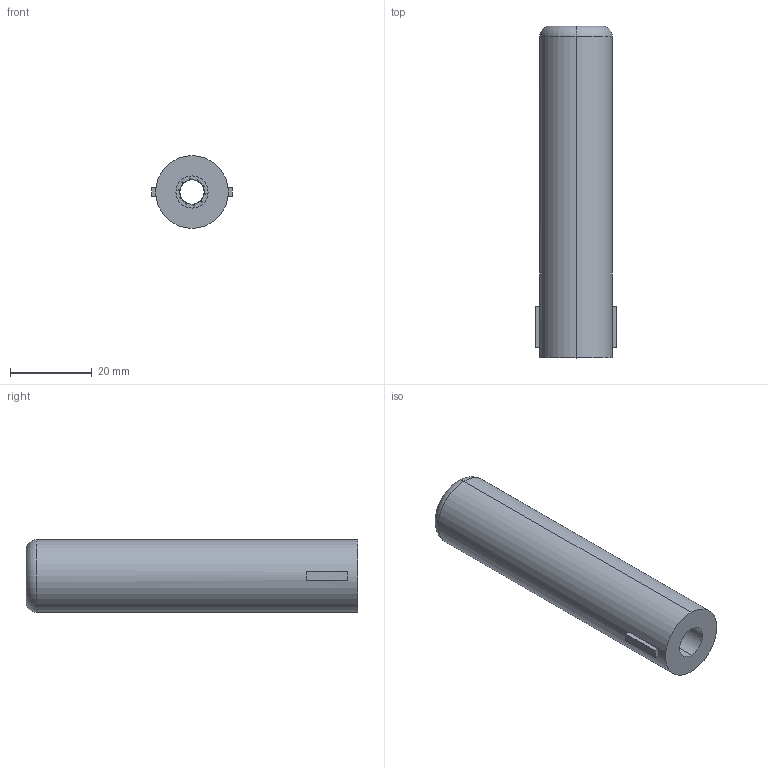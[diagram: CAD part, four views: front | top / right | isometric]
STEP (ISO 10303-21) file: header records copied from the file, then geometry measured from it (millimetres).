
FILE_DESCRIPTION (( 'STEP AP214' ), '1' );
FILE_NAME ('barrel.STEP', '2013-09-24T00:09:58', ( '' ), ( '' ), 'SwSTEP 2.0', 'SolidWorks 2013', '' );
FILE_SCHEMA (( 'AUTOMOTIVE_DESIGN' ));
Length unit declared in the file: inch
Products named in the file (1): barrel
Bounding box: 19.81 x 81.28 x 17.78 mm (x, y, z)
Volume: 17120 mm3; surface area: 7063.3 mm2
Topology: 1 solids, 1 shells, 81 faces, 226 edges, 150 vertices
Faces by surface type: cylinder 36, bspline 30, plane 13, torus 2
Entity records: 9628 total; most frequent: CARTESIAN_POINT 7878, ORIENTED_EDGE 452, DIRECTION 260, EDGE_CURVE 226, VERTEX_POINT 150, AXIS2_PLACEMENT_3D 92, EDGE_LOOP 86, ADVANCED_FACE 81
